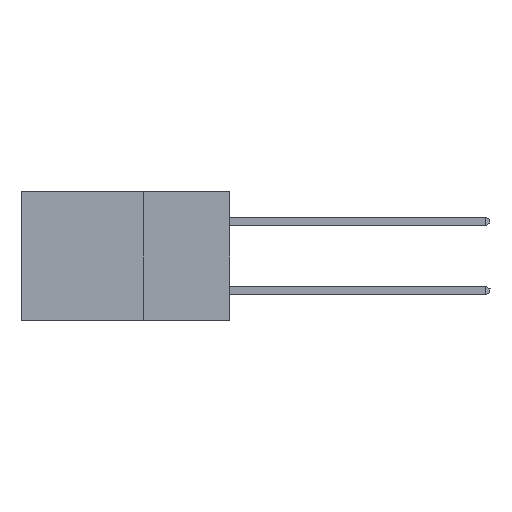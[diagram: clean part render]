
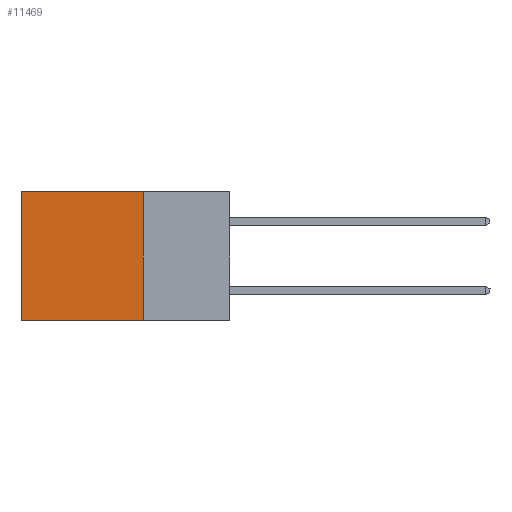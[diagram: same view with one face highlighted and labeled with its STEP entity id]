
A CAD part, left-side view. The second image highlights one B-rep face of the part: STEP entity #11469.
In plain terms, the highlighted planar face has unit normal (-1, 0, 0).
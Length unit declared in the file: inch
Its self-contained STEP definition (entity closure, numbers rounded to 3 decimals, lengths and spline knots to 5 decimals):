
#1031 = VECTOR ( 'NONE', #20693, 39.37008 ) ;
#1853 = CARTESIAN_POINT ( 'NONE',  ( 0.2615, 0.6, -0.37 ) ) ;
#2632 = ORIENTED_EDGE ( 'NONE', *, *, #7459, .T. ) ;
#2886 = CARTESIAN_POINT ( 'NONE',  ( 0.2615, 0.6, 0. ) ) ;
#2976 = PLANE ( 'NONE',  #5579 ) ;
#3267 = VERTEX_POINT ( 'NONE', #1853 ) ;
#3973 = ORIENTED_EDGE ( 'NONE', *, *, #13011, .F. ) ;
#4437 = CARTESIAN_POINT ( 'NONE',  ( 0.2615, 0.6, -0.37 ) ) ;
#4896 = LINE ( 'NONE', #11874, #18740 ) ;
#5077 = VECTOR ( 'NONE', #17797, 39.37008 ) ;
#5579 = AXIS2_PLACEMENT_3D ( 'NONE', #15690, #17475, #6665 ) ;
#5909 = LINE ( 'NONE', #4437, #1031 ) ;
#6665 = DIRECTION ( 'NONE',  ( 0., 0., -1. ) ) ;
#6845 = CARTESIAN_POINT ( 'NONE',  ( 0.2615, 0.25, -0.37 ) ) ;
#6921 = VECTOR ( 'NONE', #18992, 39.37008 ) ;
#7459 = EDGE_CURVE ( 'NONE', #10225, #3267, #5909, .T. ) ;
#8020 = FACE_OUTER_BOUND ( 'NONE', #22815, .T. ) ;
#9074 = ORIENTED_EDGE ( 'NONE', *, *, #15787, .F. ) ;
#9659 = VERTEX_POINT ( 'NONE', #6845 ) ;
#10225 = VERTEX_POINT ( 'NONE', #2886 ) ;
#10335 = CARTESIAN_POINT ( 'NONE',  ( 0.2615, 0.25, 0. ) ) ;
#11469 = ADVANCED_FACE ( 'NONE', ( #8020 ), #2976, .F. ) ;
#11874 = CARTESIAN_POINT ( 'NONE',  ( 0.2615, 0.25, 0. ) ) ;
#12083 = ORIENTED_EDGE ( 'NONE', *, *, #19713, .T. ) ;
#12445 = CARTESIAN_POINT ( 'NONE',  ( 0.2615, 0.25, -0.37 ) ) ;
#12863 = VERTEX_POINT ( 'NONE', #10335 ) ;
#13011 = EDGE_CURVE ( 'NONE', #12863, #9659, #18355, .T. ) ;
#15690 = CARTESIAN_POINT ( 'NONE',  ( 0.2615, 0.25, -0.37 ) ) ;
#15787 = EDGE_CURVE ( 'NONE', #9659, #3267, #21295, .T. ) ;
#17192 = CARTESIAN_POINT ( 'NONE',  ( 0.2615, 0.25, -0.37 ) ) ;
#17475 = DIRECTION ( 'NONE',  ( 1., 0., 0. ) ) ;
#17797 = DIRECTION ( 'NONE',  ( 0., 0., -1. ) ) ;
#18355 = LINE ( 'NONE', #12445, #5077 ) ;
#18740 = VECTOR ( 'NONE', #22588, 39.37008 ) ;
#18992 = DIRECTION ( 'NONE',  ( 0., 1., 0. ) ) ;
#19713 = EDGE_CURVE ( 'NONE', #12863, #10225, #4896, .T. ) ;
#20693 = DIRECTION ( 'NONE',  ( 0., 0., -1. ) ) ;
#21295 = LINE ( 'NONE', #17192, #6921 ) ;
#22588 = DIRECTION ( 'NONE',  ( 0., 1., 0. ) ) ;
#22815 = EDGE_LOOP ( 'NONE', ( #2632, #9074, #3973, #12083 ) ) ;
